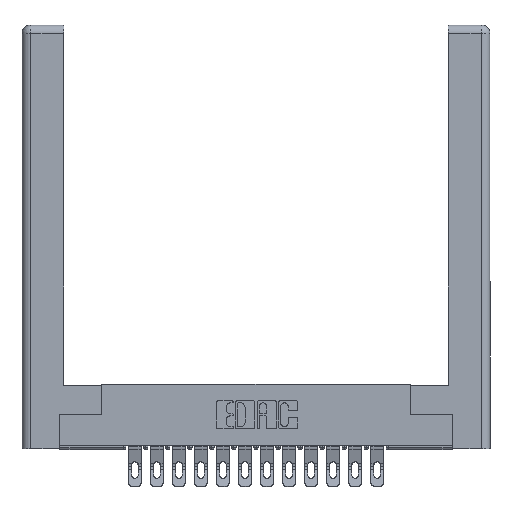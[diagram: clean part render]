
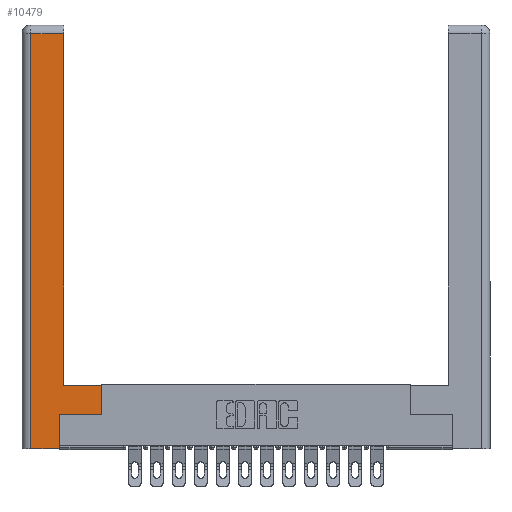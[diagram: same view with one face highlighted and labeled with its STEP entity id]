
A CAD part, top view. The second image highlights one B-rep face of the part: STEP entity #10479.
In plain terms, the highlighted planar face has unit normal (0, 0, 1).
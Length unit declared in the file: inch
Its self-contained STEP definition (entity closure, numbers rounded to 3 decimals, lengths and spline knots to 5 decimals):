
#51 = DIRECTION ( 'NONE',  ( -1., 0., 0. ) ) ;
#330 = FACE_OUTER_BOUND ( 'NONE', #14567, .T. ) ;
#493 = VERTEX_POINT ( 'NONE', #8917 ) ;
#578 = VECTOR ( 'NONE', #6390, 39.37008 ) ;
#1023 = PLANE ( 'NONE',  #4097 ) ;
#1024 = ORIENTED_EDGE ( 'NONE', *, *, #10161, .T. ) ;
#1717 = CARTESIAN_POINT ( 'NONE',  ( 0.0615, 0., 0. ) ) ;
#2421 = VERTEX_POINT ( 'NONE', #13329 ) ;
#2547 = DIRECTION ( 'NONE',  ( 0., 0., -1. ) ) ;
#2792 = ORIENTED_EDGE ( 'NONE', *, *, #9211, .T. ) ;
#2964 = LINE ( 'NONE', #1717, #578 ) ;
#3411 = DIRECTION ( 'NONE',  ( 1., 0., 0. ) ) ;
#3757 = CARTESIAN_POINT ( 'NONE',  ( 0.265, 0.245, 0. ) ) ;
#4097 = AXIS2_PLACEMENT_3D ( 'NONE', #11848, #2547, #16445 ) ;
#4194 = CARTESIAN_POINT ( 'NONE',  ( 0.295, 3., 0. ) ) ;
#4354 = CARTESIAN_POINT ( 'NONE',  ( 0.295, 0.45, 0. ) ) ;
#4363 = EDGE_CURVE ( 'NONE', #6056, #13459, #14098, .T. ) ;
#4763 = CARTESIAN_POINT ( 'NONE',  ( 0.265, 0., 0. ) ) ;
#4827 = ORIENTED_EDGE ( 'NONE', *, *, #4363, .T. ) ;
#6056 = VERTEX_POINT ( 'NONE', #15231 ) ;
#6390 = DIRECTION ( 'NONE',  ( 0., -1., 0. ) ) ;
#6483 = EDGE_CURVE ( 'NONE', #13459, #12202, #19698, .T. ) ;
#6550 = ORIENTED_EDGE ( 'NONE', *, *, #6483, .T. ) ;
#6665 = VERTEX_POINT ( 'NONE', #12344 ) ;
#6877 = DIRECTION ( 'NONE',  ( 0., 1., 0. ) ) ;
#7053 = CARTESIAN_POINT ( 'NONE',  ( 0.0615, 0., 0. ) ) ;
#7991 = EDGE_CURVE ( 'NONE', #493, #10421, #11102, .T. ) ;
#8171 = LINE ( 'NONE', #4194, #12521 ) ;
#8410 = DIRECTION ( 'NONE',  ( 1., 0., 0. ) ) ;
#8420 = CARTESIAN_POINT ( 'NONE',  ( 0.565, 0.245, 0. ) ) ;
#8467 = CARTESIAN_POINT ( 'NONE',  ( 0.565, 0.45, 0. ) ) ;
#8593 = DIRECTION ( 'NONE',  ( 0., 1., 0. ) ) ;
#8768 = VECTOR ( 'NONE', #8410, 39.37008 ) ;
#8917 = CARTESIAN_POINT ( 'NONE',  ( 0.295, 2.94, 0. ) ) ;
#9211 = EDGE_CURVE ( 'NONE', #6665, #6056, #11736, .T. ) ;
#9426 = LINE ( 'NONE', #4354, #15154 ) ;
#9622 = ORIENTED_EDGE ( 'NONE', *, *, #15352, .T. ) ;
#10111 = CARTESIAN_POINT ( 'NONE',  ( 0.0615, 2.94, 0. ) ) ;
#10161 = EDGE_CURVE ( 'NONE', #10421, #14128, #2964, .T. ) ;
#10421 = VERTEX_POINT ( 'NONE', #10111 ) ;
#10479 = ADVANCED_FACE ( 'NONE', ( #330 ), #1023, .F. ) ;
#10537 = VECTOR ( 'NONE', #6877, 39.37008 ) ;
#11102 = LINE ( 'NONE', #12125, #16299 ) ;
#11266 = CARTESIAN_POINT ( 'NONE',  ( 0.565, 0.45, 0. ) ) ;
#11736 = LINE ( 'NONE', #3757, #10537 ) ;
#11848 = CARTESIAN_POINT ( 'NONE',  ( 0., 0., 0. ) ) ;
#12123 = DIRECTION ( 'NONE',  ( 0., 1., 0. ) ) ;
#12125 = CARTESIAN_POINT ( 'NONE',  ( 0.0615, 2.94, 0. ) ) ;
#12202 = VERTEX_POINT ( 'NONE', #11266 ) ;
#12344 = CARTESIAN_POINT ( 'NONE',  ( 0.265, 0., 0. ) ) ;
#12521 = VECTOR ( 'NONE', #12123, 39.37008 ) ;
#13329 = CARTESIAN_POINT ( 'NONE',  ( 0.295, 0.45, 0. ) ) ;
#13459 = VERTEX_POINT ( 'NONE', #8420 ) ;
#13707 = LINE ( 'NONE', #4763, #18211 ) ;
#14098 = LINE ( 'NONE', #18854, #8768 ) ;
#14128 = VERTEX_POINT ( 'NONE', #7053 ) ;
#14567 = EDGE_LOOP ( 'NONE', ( #14656, #19413, #1024, #16296, #2792, #4827, #6550, #9622 ) ) ;
#14656 = ORIENTED_EDGE ( 'NONE', *, *, #15916, .T. ) ;
#15154 = VECTOR ( 'NONE', #51, 39.37008 ) ;
#15231 = CARTESIAN_POINT ( 'NONE',  ( 0.265, 0.245, 0. ) ) ;
#15352 = EDGE_CURVE ( 'NONE', #12202, #2421, #9426, .T. ) ;
#15466 = EDGE_CURVE ( 'NONE', #14128, #6665, #13707, .T. ) ;
#15916 = EDGE_CURVE ( 'NONE', #2421, #493, #8171, .T. ) ;
#16296 = ORIENTED_EDGE ( 'NONE', *, *, #15466, .T. ) ;
#16299 = VECTOR ( 'NONE', #19651, 39.37008 ) ;
#16445 = DIRECTION ( 'NONE',  ( -1., 0., 0. ) ) ;
#18211 = VECTOR ( 'NONE', #3411, 39.37008 ) ;
#18473 = VECTOR ( 'NONE', #8593, 39.37008 ) ;
#18854 = CARTESIAN_POINT ( 'NONE',  ( 0.565, 0.245, 0. ) ) ;
#19413 = ORIENTED_EDGE ( 'NONE', *, *, #7991, .T. ) ;
#19651 = DIRECTION ( 'NONE',  ( -1., 0., 0. ) ) ;
#19698 = LINE ( 'NONE', #8467, #18473 ) ;
